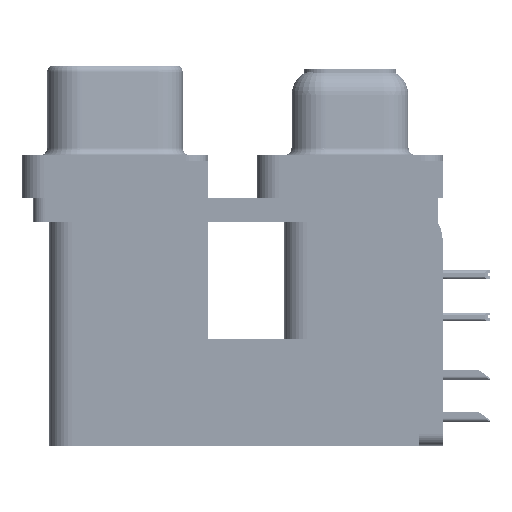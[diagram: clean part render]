
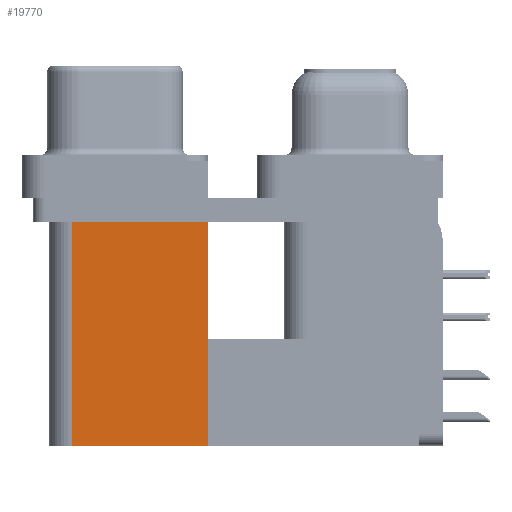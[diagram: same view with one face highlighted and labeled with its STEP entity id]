
A CAD part, left-side view. The second image highlights one B-rep face of the part: STEP entity #19770.
In plain terms, the highlighted planar face has unit normal (-1, 0, 0).
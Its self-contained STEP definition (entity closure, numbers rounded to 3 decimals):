
#2265 = EDGE_CURVE ( 'NONE', #16102, #5772, #48780, .T. ) ;
#5772 = VERTEX_POINT ( 'NONE', #52713 ) ;
#7304 = FACE_OUTER_BOUND ( 'NONE', #52855, .T. ) ;
#10707 = EDGE_CURVE ( 'NONE', #47657, #5772, #14592, .T. ) ;
#12956 = CARTESIAN_POINT ( 'NONE',  ( 3.7, 18.8, -19.2 ) ) ;
#13337 = VERTEX_POINT ( 'NONE', #46250 ) ;
#14449 = DIRECTION ( 'NONE',  ( 0., 0., 1. ) ) ;
#14592 = LINE ( 'NONE', #47409, #24561 ) ;
#15944 = EDGE_CURVE ( 'NONE', #13337, #47657, #28235, .T. ) ;
#16102 = VERTEX_POINT ( 'NONE', #39840 ) ;
#19770 = ADVANCED_FACE ( 'NONE', ( #7304 ), #28705, .F. ) ;
#21333 = ORIENTED_EDGE ( 'NONE', *, *, #2265, .T. ) ;
#24561 = VECTOR ( 'NONE', #43495, 1000. ) ;
#26830 = ORIENTED_EDGE ( 'NONE', *, *, #15944, .F. ) ;
#27162 = DIRECTION ( 'NONE',  ( 0., 1., 0. ) ) ;
#28235 = LINE ( 'NONE', #45165, #35228 ) ;
#28705 = PLANE ( 'NONE',  #42590 ) ;
#29636 = EDGE_CURVE ( 'NONE', #13337, #16102, #51691, .T. ) ;
#30061 = VECTOR ( 'NONE', #27162, 1000. ) ;
#33697 = DIRECTION ( 'NONE',  ( 0., 0., -1. ) ) ;
#34363 = VECTOR ( 'NONE', #14449, 1000. ) ;
#35228 = VECTOR ( 'NONE', #36835, 1000. ) ;
#36835 = DIRECTION ( 'NONE',  ( 0., 1., 0. ) ) ;
#37021 = ORIENTED_EDGE ( 'NONE', *, *, #10707, .F. ) ;
#37544 = ORIENTED_EDGE ( 'NONE', *, *, #29636, .T. ) ;
#39840 = CARTESIAN_POINT ( 'NONE',  ( 3.7, 9.6, -2.5 ) ) ;
#42590 = AXIS2_PLACEMENT_3D ( 'NONE', #54498, #46183, #33697 ) ;
#43495 = DIRECTION ( 'NONE',  ( 0., 0., 1. ) ) ;
#44700 = CARTESIAN_POINT ( 'NONE',  ( 3.7, 9.6, -19.2 ) ) ;
#45165 = CARTESIAN_POINT ( 'NONE',  ( 3.7, 9.6, -19.2 ) ) ;
#46183 = DIRECTION ( 'NONE',  ( 1., 0., 0. ) ) ;
#46250 = CARTESIAN_POINT ( 'NONE',  ( 3.7, 9.6, -19.2 ) ) ;
#47409 = CARTESIAN_POINT ( 'NONE',  ( 3.7, 18.8, -19.2 ) ) ;
#47657 = VERTEX_POINT ( 'NONE', #12956 ) ;
#48780 = LINE ( 'NONE', #53497, #30061 ) ;
#51691 = LINE ( 'NONE', #44700, #34363 ) ;
#52713 = CARTESIAN_POINT ( 'NONE',  ( 3.7, 18.8, -2.5 ) ) ;
#52855 = EDGE_LOOP ( 'NONE', ( #21333, #37021, #26830, #37544 ) ) ;
#53497 = CARTESIAN_POINT ( 'NONE',  ( 3.7, 9.6, -2.5 ) ) ;
#54498 = CARTESIAN_POINT ( 'NONE',  ( 3.7, 9.6, -19.2 ) ) ;
